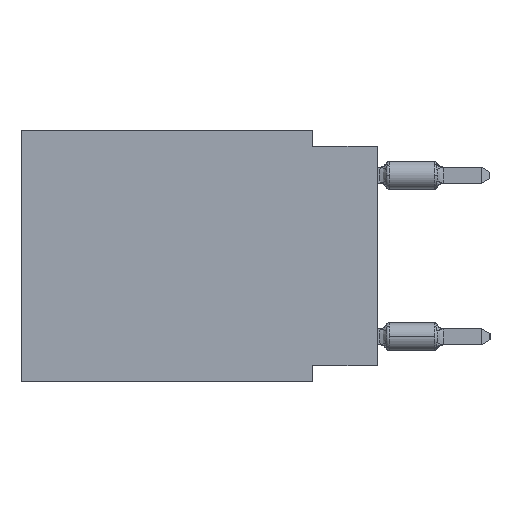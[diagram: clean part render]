
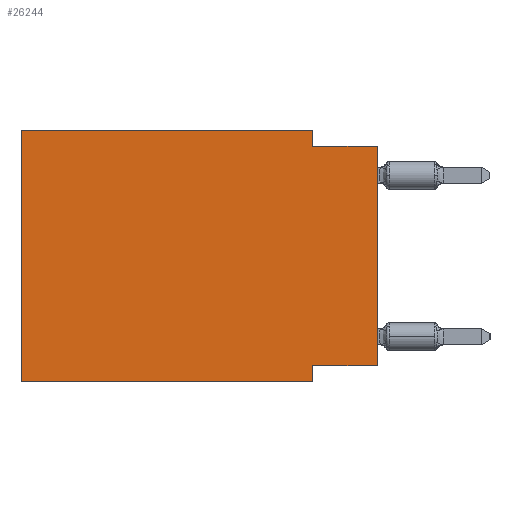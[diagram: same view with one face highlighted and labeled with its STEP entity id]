
A CAD part, left-side view. The second image highlights one B-rep face of the part: STEP entity #26244.
In plain terms, the highlighted planar face has unit normal (-1, 0, 0).
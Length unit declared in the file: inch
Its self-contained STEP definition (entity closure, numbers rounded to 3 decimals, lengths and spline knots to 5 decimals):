
#1704 = DIRECTION ( 'NONE',  ( 0., -1., 0. ) ) ;
#2128 = VECTOR ( 'NONE', #29549, 39.37008 ) ;
#3602 = CARTESIAN_POINT ( 'NONE',  ( 0., 0.1, -0.39 ) ) ;
#3865 = CARTESIAN_POINT ( 'NONE',  ( 0., 0.55, 0. ) ) ;
#4679 = EDGE_CURVE ( 'NONE', #32140, #37145, #6440, .T. ) ;
#5408 = CARTESIAN_POINT ( 'NONE',  ( 0., 0.1, -0.365 ) ) ;
#6440 = LINE ( 'NONE', #43939, #19664 ) ;
#6619 = DIRECTION ( 'NONE',  ( 0., 0., 1. ) ) ;
#6656 = VERTEX_POINT ( 'NONE', #3865 ) ;
#8315 = CARTESIAN_POINT ( 'NONE',  ( 0., 0., -0.365 ) ) ;
#10187 = EDGE_CURVE ( 'NONE', #38391, #15970, #30535, .T. ) ;
#10349 = CARTESIAN_POINT ( 'NONE',  ( 0., 0., 0. ) ) ;
#11945 = VECTOR ( 'NONE', #31379, 39.37008 ) ;
#12371 = EDGE_CURVE ( 'NONE', #6656, #36438, #26780, .T. ) ;
#12855 = ORIENTED_EDGE ( 'NONE', *, *, #28143, .T. ) ;
#15970 = VERTEX_POINT ( 'NONE', #5408 ) ;
#16392 = CARTESIAN_POINT ( 'NONE',  ( 0., 0.55, -0.39 ) ) ;
#17016 = DIRECTION ( 'NONE',  ( 0., 0., -1. ) ) ;
#18790 = DIRECTION ( 'NONE',  ( 0., -1., 0. ) ) ;
#18951 = DIRECTION ( 'NONE',  ( 0., 0., -1. ) ) ;
#19195 = ORIENTED_EDGE ( 'NONE', *, *, #10187, .F. ) ;
#19329 = EDGE_CURVE ( 'NONE', #37449, #6656, #29074, .T. ) ;
#19664 = VECTOR ( 'NONE', #1704, 39.37008 ) ;
#20753 = AXIS2_PLACEMENT_3D ( 'NONE', #24595, #47629, #21603 ) ;
#21250 = LINE ( 'NONE', #21489, #28131 ) ;
#21481 = ORIENTED_EDGE ( 'NONE', *, *, #42329, .F. ) ;
#21489 = CARTESIAN_POINT ( 'NONE',  ( 0., 0.1, -0.39 ) ) ;
#21603 = DIRECTION ( 'NONE',  ( 0., 0., -1. ) ) ;
#21693 = VECTOR ( 'NONE', #6619, 39.37008 ) ;
#23041 = CARTESIAN_POINT ( 'NONE',  ( 0., 0.1, -0.025 ) ) ;
#23643 = LINE ( 'NONE', #16392, #11945 ) ;
#24595 = CARTESIAN_POINT ( 'NONE',  ( 0., 0.55, 0. ) ) ;
#24817 = EDGE_CURVE ( 'NONE', #37449, #28297, #23643, .T. ) ;
#25342 = FACE_OUTER_BOUND ( 'NONE', #38629, .T. ) ;
#25436 = ORIENTED_EDGE ( 'NONE', *, *, #44807, .F. ) ;
#25541 = CARTESIAN_POINT ( 'NONE',  ( 0., 0., -0.025 ) ) ;
#25564 = VECTOR ( 'NONE', #27286, 39.37008 ) ;
#25718 = LINE ( 'NONE', #44724, #37880 ) ;
#25973 = CARTESIAN_POINT ( 'NONE',  ( 0., 0.55, -0.39 ) ) ;
#26244 = ADVANCED_FACE ( 'NONE', ( #25342 ), #39865, .F. ) ;
#26780 = LINE ( 'NONE', #38554, #43292 ) ;
#27286 = DIRECTION ( 'NONE',  ( 0., 1., 0. ) ) ;
#28131 = VECTOR ( 'NONE', #17016, 39.37008 ) ;
#28143 = EDGE_CURVE ( 'NONE', #38391, #37145, #45102, .T. ) ;
#28297 = VERTEX_POINT ( 'NONE', #3602 ) ;
#28819 = CARTESIAN_POINT ( 'NONE',  ( 0., 0.55, 0. ) ) ;
#29074 = LINE ( 'NONE', #28819, #2128 ) ;
#29549 = DIRECTION ( 'NONE',  ( 0., 0., 1. ) ) ;
#30534 = CARTESIAN_POINT ( 'NONE',  ( 0., 0., -0.365 ) ) ;
#30535 = LINE ( 'NONE', #8315, #25564 ) ;
#31379 = DIRECTION ( 'NONE',  ( 0., -1., 0. ) ) ;
#32140 = VERTEX_POINT ( 'NONE', #23041 ) ;
#33558 = ORIENTED_EDGE ( 'NONE', *, *, #12371, .F. ) ;
#36438 = VERTEX_POINT ( 'NONE', #38911 ) ;
#37145 = VERTEX_POINT ( 'NONE', #25541 ) ;
#37449 = VERTEX_POINT ( 'NONE', #25973 ) ;
#37880 = VECTOR ( 'NONE', #18951, 39.37008 ) ;
#38391 = VERTEX_POINT ( 'NONE', #30534 ) ;
#38554 = CARTESIAN_POINT ( 'NONE',  ( 0., 0.55, 0. ) ) ;
#38629 = EDGE_LOOP ( 'NONE', ( #12855, #45227, #25436, #33558, #47123, #46346, #21481, #19195 ) ) ;
#38911 = CARTESIAN_POINT ( 'NONE',  ( 0., 0.1, 0. ) ) ;
#39865 = PLANE ( 'NONE',  #20753 ) ;
#42329 = EDGE_CURVE ( 'NONE', #15970, #28297, #21250, .T. ) ;
#43292 = VECTOR ( 'NONE', #18790, 39.37008 ) ;
#43939 = CARTESIAN_POINT ( 'NONE',  ( 0., 0., -0.025 ) ) ;
#44724 = CARTESIAN_POINT ( 'NONE',  ( 0., 0.1, 0. ) ) ;
#44807 = EDGE_CURVE ( 'NONE', #36438, #32140, #25718, .T. ) ;
#45102 = LINE ( 'NONE', #10349, #21693 ) ;
#45227 = ORIENTED_EDGE ( 'NONE', *, *, #4679, .F. ) ;
#46346 = ORIENTED_EDGE ( 'NONE', *, *, #24817, .T. ) ;
#47123 = ORIENTED_EDGE ( 'NONE', *, *, #19329, .F. ) ;
#47629 = DIRECTION ( 'NONE',  ( 1., 0., 0. ) ) ;
